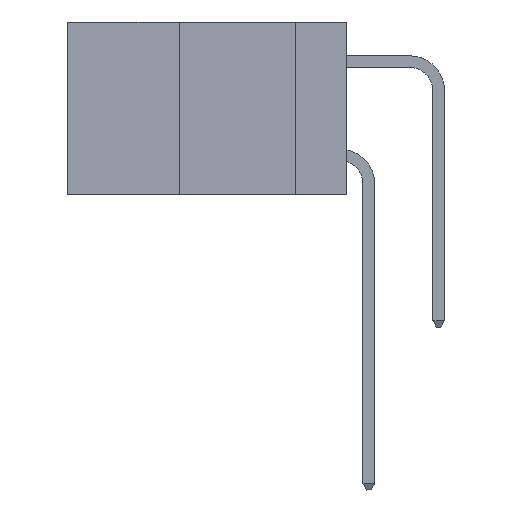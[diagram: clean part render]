
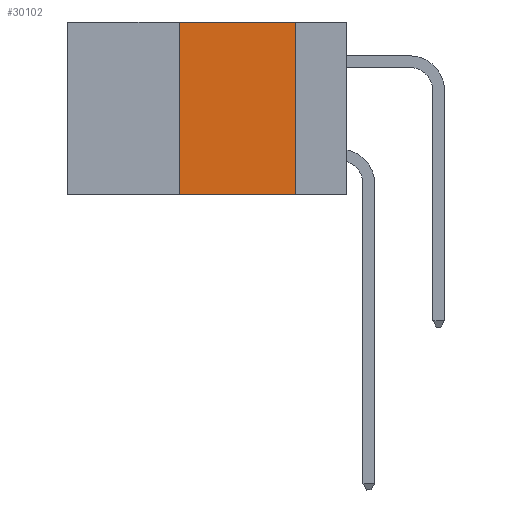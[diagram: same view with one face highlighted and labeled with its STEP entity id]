
A CAD part, left-side view. The second image highlights one B-rep face of the part: STEP entity #30102.
In plain terms, the highlighted planar face has unit normal (-1, 0, 0).
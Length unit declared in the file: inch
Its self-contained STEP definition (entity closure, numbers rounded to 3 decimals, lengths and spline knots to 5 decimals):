
#171 = CARTESIAN_POINT ( 'NONE',  ( 0., 0.36, -0.37 ) ) ;
#2717 = CARTESIAN_POINT ( 'NONE',  ( 0., 0.6, -0.37 ) ) ;
#2777 = CARTESIAN_POINT ( 'NONE',  ( 0., 0.11, 0. ) ) ;
#2867 = DIRECTION ( 'NONE',  ( 1., 0., 0. ) ) ;
#5542 = VECTOR ( 'NONE', #22449, 39.37008 ) ;
#10489 = EDGE_CURVE ( 'NONE', #35101, #30257, #13205, .T. ) ;
#13189 = VECTOR ( 'NONE', #29197, 39.37008 ) ;
#13205 = LINE ( 'NONE', #25501, #15194 ) ;
#14957 = EDGE_CURVE ( 'NONE', #30257, #18616, #31387, .T. ) ;
#15194 = VECTOR ( 'NONE', #36756, 39.37008 ) ;
#16525 = CARTESIAN_POINT ( 'NONE',  ( 0., 0.36, 0. ) ) ;
#17662 = PLANE ( 'NONE',  #18580 ) ;
#18580 = AXIS2_PLACEMENT_3D ( 'NONE', #29528, #2867, #26633 ) ;
#18616 = VERTEX_POINT ( 'NONE', #20475 ) ;
#18731 = EDGE_LOOP ( 'NONE', ( #29874, #36105, #33758, #29988 ) ) ;
#19330 = CARTESIAN_POINT ( 'NONE',  ( 0., 0.6, 0. ) ) ;
#20051 = LINE ( 'NONE', #2717, #13189 ) ;
#20436 = EDGE_CURVE ( 'NONE', #35101, #31940, #20051, .T. ) ;
#20475 = CARTESIAN_POINT ( 'NONE',  ( 0., 0.11, 0. ) ) ;
#22091 = CARTESIAN_POINT ( 'NONE',  ( 0., 0.11, -0.37 ) ) ;
#22449 = DIRECTION ( 'NONE',  ( 0., -1., 0. ) ) ;
#23792 = DIRECTION ( 'NONE',  ( 0., 0., -1. ) ) ;
#25501 = CARTESIAN_POINT ( 'NONE',  ( 0., 0.36, 0. ) ) ;
#26633 = DIRECTION ( 'NONE',  ( 0., 0., -1. ) ) ;
#28503 = LINE ( 'NONE', #2777, #31695 ) ;
#29197 = DIRECTION ( 'NONE',  ( 0., -1., 0. ) ) ;
#29528 = CARTESIAN_POINT ( 'NONE',  ( 0., 0.6, 0. ) ) ;
#29874 = ORIENTED_EDGE ( 'NONE', *, *, #30892, .F. ) ;
#29988 = ORIENTED_EDGE ( 'NONE', *, *, #20436, .T. ) ;
#30102 = ADVANCED_FACE ( 'NONE', ( #32447 ), #17662, .F. ) ;
#30257 = VERTEX_POINT ( 'NONE', #16525 ) ;
#30892 = EDGE_CURVE ( 'NONE', #18616, #31940, #28503, .T. ) ;
#31387 = LINE ( 'NONE', #19330, #5542 ) ;
#31695 = VECTOR ( 'NONE', #23792, 39.37008 ) ;
#31940 = VERTEX_POINT ( 'NONE', #22091 ) ;
#32447 = FACE_OUTER_BOUND ( 'NONE', #18731, .T. ) ;
#33758 = ORIENTED_EDGE ( 'NONE', *, *, #10489, .F. ) ;
#35101 = VERTEX_POINT ( 'NONE', #171 ) ;
#36105 = ORIENTED_EDGE ( 'NONE', *, *, #14957, .F. ) ;
#36756 = DIRECTION ( 'NONE',  ( 0., 0., 1. ) ) ;
